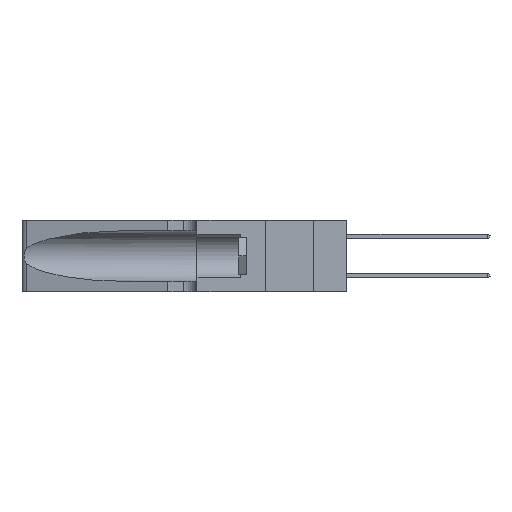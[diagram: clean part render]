
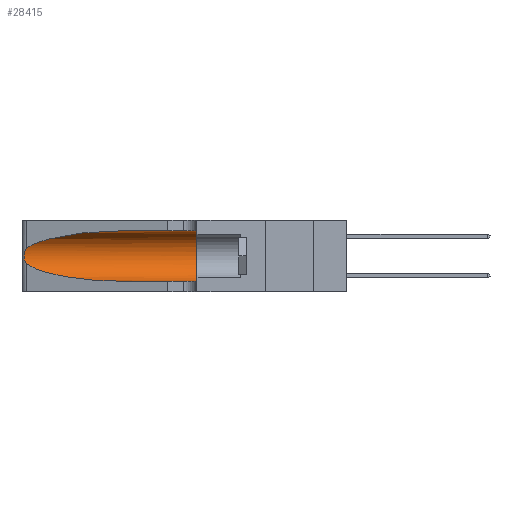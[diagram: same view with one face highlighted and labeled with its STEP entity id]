
A CAD part, left-side view. The second image highlights one B-rep face of the part: STEP entity #28415.
In plain terms, the highlighted cylindrical face has radius 3.308 mm (diameter 6.617 mm), a partial arc.
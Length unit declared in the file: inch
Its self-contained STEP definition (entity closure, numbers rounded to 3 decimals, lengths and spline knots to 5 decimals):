
#562 = VERTEX_POINT ( 'NONE', #31014 ) ;
#685 = CARTESIAN_POINT ( 'NONE',  ( 0.1305, 0.72297, 0.31525 ) ) ;
#2145 = DIRECTION ( 'NONE',  ( 0., -1., 0. ) ) ;
#3058 = CARTESIAN_POINT ( 'NONE',  ( 0.18966, 0.96281, 0.31525 ) ) ;
#3873 = CARTESIAN_POINT ( 'NONE',  ( 0.26018, 1.23835, 0.19895 ) ) ;
#4557 = EDGE_CURVE ( 'NONE', #46501, #32714, #26656, .T. ) ;
#5829 = CARTESIAN_POINT ( 'NONE',  ( 0.25487, 1.22718, 0.22369 ) ) ;
#5950 = B_SPLINE_CURVE_WITH_KNOTS ( 'NONE', 3,
 ( #41479, #45096, #27083, #42989, #25981, #3873, #29673, #7613, #33294, #11355, #36938, #15057, #40550, #18768 ),
 .UNSPECIFIED., .F., .F.,
 ( 4, 2, 2, 2, 2, 2, 4 ),
 ( 0., 0.00027, 0.00053, 0.00107, 0.0016, 0.00187, 0.00214 ),
 .UNSPECIFIED. ) ;
#5987 = CARTESIAN_POINT ( 'NONE',  ( 0.1305, 1.61858, 0.05475 ) ) ;
#6439 = CARTESIAN_POINT ( 'NONE',  ( 0.25487, 1.22718, 0.14631 ) ) ;
#6797 = CARTESIAN_POINT ( 'NONE',  ( 0.2373, 1.15595, 0.28018 ) ) ;
#6848 = DIRECTION ( 'NONE',  ( 0., 1., 0. ) ) ;
#7613 = CARTESIAN_POINT ( 'NONE',  ( 0.26075, 1.23896, 0.178 ) ) ;
#9024 = ORIENTED_EDGE ( 'NONE', *, *, #33242, .T. ) ;
#10144 = CARTESIAN_POINT ( 'NONE',  ( 0.2373, 1.15595, 0.08982 ) ) ;
#10514 = CARTESIAN_POINT ( 'NONE',  ( 0.1305, 0.72297, 0.31525 ) ) ;
#11195 = FACE_OUTER_BOUND ( 'NONE', #25641, .T. ) ;
#11355 = CARTESIAN_POINT ( 'NONE',  ( 0.25856, 1.23593, 0.16098 ) ) ;
#13156 = CARTESIAN_POINT ( 'NONE',  ( 0.1305, 0.35, 0.05475 ) ) ;
#13827 = EDGE_CURVE ( 'NONE', #46501, #29243, #18443, .T. ) ;
#13880 = CARTESIAN_POINT ( 'NONE',  ( 0.1305, 0.72297, 0.05475 ) ) ;
#15057 = CARTESIAN_POINT ( 'NONE',  ( 0.25639, 1.23186, 0.15144 ) ) ;
#15526 = VERTEX_POINT ( 'NONE', #13156 ) ;
#16473 = AXIS2_PLACEMENT_3D ( 'NONE', #19434, #23095, #30465 ) ;
#18332 = EDGE_CURVE ( 'NONE', #562, #15526, #23429, .T. ) ;
#18443 = LINE ( 'NONE', #24277, #45161 ) ;
#18768 = CARTESIAN_POINT ( 'NONE',  ( 0.25487, 1.22718, 0.14631 ) ) ;
#18884 = CARTESIAN_POINT ( 'NONE',  ( 0.25487, 1.22718, 0.14631 ) ) ;
#19434 = CARTESIAN_POINT ( 'NONE',  ( 0.1305, 1.61858, 0.185 ) ) ;
#20747 = ORIENTED_EDGE ( 'NONE', *, *, #33728, .T. ) ;
#22775 = ORIENTED_EDGE ( 'NONE', *, *, #18332, .T. ) ;
#23095 = DIRECTION ( 'NONE',  ( 0., -1., 0. ) ) ;
#23429 = LINE ( 'NONE', #5987, #41605 ) ;
#24277 = CARTESIAN_POINT ( 'NONE',  ( 0.1305, 1.61858, 0.31525 ) ) ;
#24798 = CARTESIAN_POINT ( 'NONE',  ( 0.1305, 0.35, 0.31525 ) ) ;
#25641 = EDGE_LOOP ( 'NONE', ( #27095, #9024, #20747, #22775, #43397, #36367 ) ) ;
#25981 = CARTESIAN_POINT ( 'NONE',  ( 0.25854, 1.2359, 0.20912 ) ) ;
#26656 =( BOUNDED_CURVE ( )  B_SPLINE_CURVE ( 3, ( #10514, #3058, #6797, #36136 ),
 .UNSPECIFIED., .F., .F. ) 
 B_SPLINE_CURVE_WITH_KNOTS ( ( 4, 4 ),
 ( 1.5708, 2.84003 ),
 .UNSPECIFIED. ) 
 CURVE ( )  GEOMETRIC_REPRESENTATION_ITEM ( )  RATIONAL_B_SPLINE_CURVE ( ( 1., 0.87, 0.87, 1. ) ) 
 REPRESENTATION_ITEM ( '' )  );
#27083 = CARTESIAN_POINT ( 'NONE',  ( 0.25639, 1.23184, 0.21858 ) ) ;
#27095 = ORIENTED_EDGE ( 'NONE', *, *, #4557, .T. ) ;
#28415 = ADVANCED_FACE ( 'NONE', ( #11195 ), #46515, .F. ) ;
#28906 = CARTESIAN_POINT ( 'NONE',  ( 0.1305, 0.35, 0.185 ) ) ;
#29243 = VERTEX_POINT ( 'NONE', #24798 ) ;
#29673 = CARTESIAN_POINT ( 'NONE',  ( 0.26075, 1.23896, 0.19203 ) ) ;
#30465 = DIRECTION ( 'NONE',  ( 0., 0., -1. ) ) ;
#31014 = CARTESIAN_POINT ( 'NONE',  ( 0.1305, 0.72297, 0.05475 ) ) ;
#31864 = DIRECTION ( 'NONE',  ( 0., -1., 0. ) ) ;
#32566 = DIRECTION ( 'NONE',  ( 0., 0., 1. ) ) ;
#32714 = VERTEX_POINT ( 'NONE', #5829 ) ;
#33242 = EDGE_CURVE ( 'NONE', #32714, #35885, #5950, .T. ) ;
#33294 = CARTESIAN_POINT ( 'NONE',  ( 0.26017, 1.23833, 0.17102 ) ) ;
#33728 = EDGE_CURVE ( 'NONE', #35885, #562, #44911, .T. ) ;
#35783 = CARTESIAN_POINT ( 'NONE',  ( 0.18966, 0.96281, 0.05475 ) ) ;
#35885 = VERTEX_POINT ( 'NONE', #18884 ) ;
#36136 = CARTESIAN_POINT ( 'NONE',  ( 0.25487, 1.22718, 0.22369 ) ) ;
#36367 = ORIENTED_EDGE ( 'NONE', *, *, #13827, .F. ) ;
#36938 = CARTESIAN_POINT ( 'NONE',  ( 0.25789, 1.23486, 0.15765 ) ) ;
#37898 = AXIS2_PLACEMENT_3D ( 'NONE', #28906, #6848, #32566 ) ;
#40550 = CARTESIAN_POINT ( 'NONE',  ( 0.25555, 1.22993, 0.14849 ) ) ;
#41080 = CIRCLE ( 'NONE', #37898, 0.13025 ) ;
#41479 = CARTESIAN_POINT ( 'NONE',  ( 0.25487, 1.22718, 0.22369 ) ) ;
#41605 = VECTOR ( 'NONE', #31864, 39.37008 ) ;
#41993 = EDGE_CURVE ( 'NONE', #29243, #15526, #41080, .T. ) ;
#42989 = CARTESIAN_POINT ( 'NONE',  ( 0.25787, 1.23484, 0.2124 ) ) ;
#43397 = ORIENTED_EDGE ( 'NONE', *, *, #41993, .F. ) ;
#44911 =( BOUNDED_CURVE ( )  B_SPLINE_CURVE ( 3, ( #6439, #10144, #35783, #13880 ),
 .UNSPECIFIED., .F., .F. ) 
 B_SPLINE_CURVE_WITH_KNOTS ( ( 4, 4 ),
 ( 3.44316, 4.71239 ),
 .UNSPECIFIED. ) 
 CURVE ( )  GEOMETRIC_REPRESENTATION_ITEM ( )  RATIONAL_B_SPLINE_CURVE ( ( 1., 0.87, 0.87, 1. ) ) 
 REPRESENTATION_ITEM ( '' )  );
#45096 = CARTESIAN_POINT ( 'NONE',  ( 0.25555, 1.22994, 0.2215 ) ) ;
#45161 = VECTOR ( 'NONE', #2145, 39.37008 ) ;
#46501 = VERTEX_POINT ( 'NONE', #685 ) ;
#46515 = CYLINDRICAL_SURFACE ( 'NONE', #16473, 0.13025 ) ;
